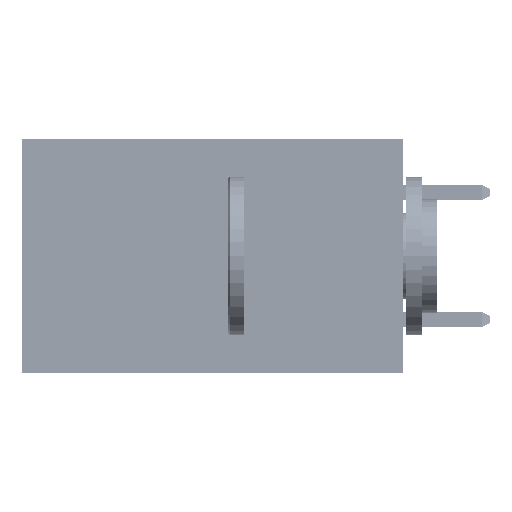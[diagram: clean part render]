
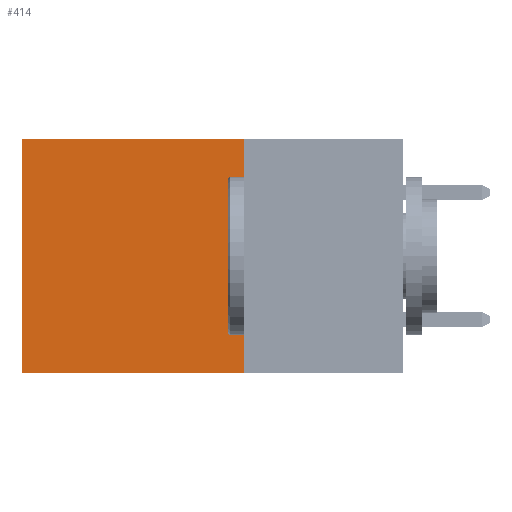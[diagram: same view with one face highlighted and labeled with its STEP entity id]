
A CAD part, left-side view. The second image highlights one B-rep face of the part: STEP entity #414.
In plain terms, the highlighted planar face has unit normal (-1, 0, 0).
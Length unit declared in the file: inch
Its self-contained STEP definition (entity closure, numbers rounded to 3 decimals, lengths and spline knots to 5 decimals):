
#389 = DIRECTION ( 'NONE',  ( 0., 0., -1. ) ) ;
#414 = ADVANCED_FACE ( 'NONE', ( #19898 ), #18087, .F. ) ;
#1550 = CARTESIAN_POINT ( 'NONE',  ( 0.2875, 0.6, 0. ) ) ;
#1611 = CARTESIAN_POINT ( 'NONE',  ( 0.2875, 0.25, 0. ) ) ;
#1769 = VECTOR ( 'NONE', #23887, 39.37008 ) ;
#2167 = LINE ( 'NONE', #36650, #40395 ) ;
#2742 = EDGE_CURVE ( 'NONE', #22773, #15125, #2167, .T. ) ;
#3833 = ORIENTED_EDGE ( 'NONE', *, *, #2742, .F. ) ;
#5261 = AXIS2_PLACEMENT_3D ( 'NONE', #32328, #32502, #43923 ) ;
#6669 = EDGE_CURVE ( 'NONE', #15125, #20111, #12873, .T. ) ;
#7455 = VERTEX_POINT ( 'NONE', #46882 ) ;
#10701 = VECTOR ( 'NONE', #35532, 39.37008 ) ;
#12873 = LINE ( 'NONE', #23398, #1769 ) ;
#15125 = VERTEX_POINT ( 'NONE', #36045 ) ;
#15232 = EDGE_LOOP ( 'NONE', ( #19388, #36609, #3833, #44807 ) ) ;
#16496 = CARTESIAN_POINT ( 'NONE',  ( 0.2875, 0.25, 0. ) ) ;
#17187 = LINE ( 'NONE', #1611, #18362 ) ;
#18087 = PLANE ( 'NONE',  #5261 ) ;
#18362 = VECTOR ( 'NONE', #27573, 39.37008 ) ;
#19388 = ORIENTED_EDGE ( 'NONE', *, *, #46965, .T. ) ;
#19898 = FACE_OUTER_BOUND ( 'NONE', #15232, .T. ) ;
#20111 = VERTEX_POINT ( 'NONE', #39147 ) ;
#21764 = LINE ( 'NONE', #1550, #10701 ) ;
#22773 = VERTEX_POINT ( 'NONE', #16496 ) ;
#23398 = CARTESIAN_POINT ( 'NONE',  ( 0.2875, 0.25, -0.37 ) ) ;
#23887 = DIRECTION ( 'NONE',  ( 0., 1., 0. ) ) ;
#27573 = DIRECTION ( 'NONE',  ( 0., 1., 0. ) ) ;
#32328 = CARTESIAN_POINT ( 'NONE',  ( 0.2875, 0.25, 0. ) ) ;
#32502 = DIRECTION ( 'NONE',  ( 1., 0., 0. ) ) ;
#32911 = EDGE_CURVE ( 'NONE', #22773, #7455, #17187, .T. ) ;
#35532 = DIRECTION ( 'NONE',  ( 0., 0., -1. ) ) ;
#36045 = CARTESIAN_POINT ( 'NONE',  ( 0.2875, 0.25, -0.37 ) ) ;
#36609 = ORIENTED_EDGE ( 'NONE', *, *, #6669, .F. ) ;
#36650 = CARTESIAN_POINT ( 'NONE',  ( 0.2875, 0.25, 0. ) ) ;
#39147 = CARTESIAN_POINT ( 'NONE',  ( 0.2875, 0.6, -0.37 ) ) ;
#40395 = VECTOR ( 'NONE', #389, 39.37008 ) ;
#43923 = DIRECTION ( 'NONE',  ( 0., 0., -1. ) ) ;
#44807 = ORIENTED_EDGE ( 'NONE', *, *, #32911, .T. ) ;
#46882 = CARTESIAN_POINT ( 'NONE',  ( 0.2875, 0.6, 0. ) ) ;
#46965 = EDGE_CURVE ( 'NONE', #7455, #20111, #21764, .T. ) ;
